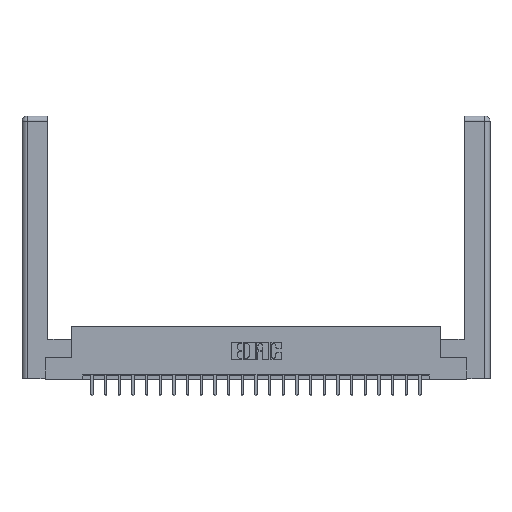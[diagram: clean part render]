
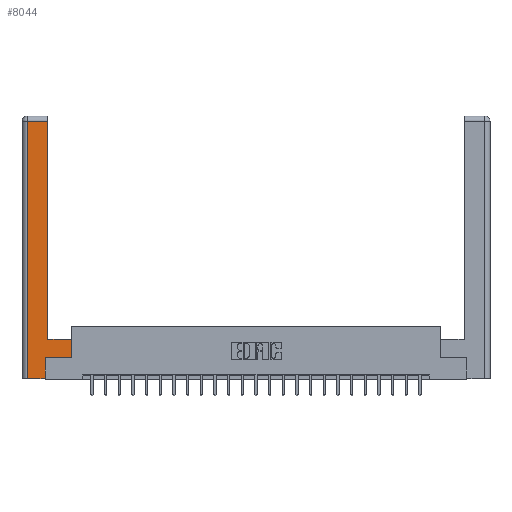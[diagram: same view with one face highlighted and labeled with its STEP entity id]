
A CAD part, top view. The second image highlights one B-rep face of the part: STEP entity #8044.
In plain terms, the highlighted planar face has unit normal (0, 0, 1).
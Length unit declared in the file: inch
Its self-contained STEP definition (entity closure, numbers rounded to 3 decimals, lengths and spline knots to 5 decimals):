
#282 = EDGE_LOOP ( 'NONE', ( #10034, #5375, #18630, #16974, #4671, #824, #2832, #15656 ) ) ;
#824 = ORIENTED_EDGE ( 'NONE', *, *, #4130, .T. ) ;
#983 = CARTESIAN_POINT ( 'NONE',  ( 0.0615, 0., 0. ) ) ;
#1534 = EDGE_CURVE ( 'NONE', #4164, #9989, #23469, .T. ) ;
#1827 = CARTESIAN_POINT ( 'NONE',  ( 0.295, 0.45, 0. ) ) ;
#1975 = FACE_OUTER_BOUND ( 'NONE', #282, .T. ) ;
#2264 = CARTESIAN_POINT ( 'NONE',  ( 0.565, 0.45, 0. ) ) ;
#2832 = ORIENTED_EDGE ( 'NONE', *, *, #22655, .T. ) ;
#2943 = CARTESIAN_POINT ( 'NONE',  ( 0., 0., 0. ) ) ;
#3510 = LINE ( 'NONE', #2264, #11119 ) ;
#4028 = CARTESIAN_POINT ( 'NONE',  ( 0.565, 0.245, 0. ) ) ;
#4130 = EDGE_CURVE ( 'NONE', #22083, #5999, #19548, .T. ) ;
#4164 = VERTEX_POINT ( 'NONE', #24257 ) ;
#4671 = ORIENTED_EDGE ( 'NONE', *, *, #22388, .T. ) ;
#4868 = VECTOR ( 'NONE', #6932, 39.37008 ) ;
#5162 = DIRECTION ( 'NONE',  ( 1., 0., 0. ) ) ;
#5306 = CARTESIAN_POINT ( 'NONE',  ( 0.0615, 2.94, 0. ) ) ;
#5375 = ORIENTED_EDGE ( 'NONE', *, *, #24340, .T. ) ;
#5926 = DIRECTION ( 'NONE',  ( 0., 1., 0. ) ) ;
#5999 = VERTEX_POINT ( 'NONE', #4028 ) ;
#6002 = VERTEX_POINT ( 'NONE', #6073 ) ;
#6073 = CARTESIAN_POINT ( 'NONE',  ( 0.295, 2.94, 0. ) ) ;
#6134 = VERTEX_POINT ( 'NONE', #21155 ) ;
#6441 = LINE ( 'NONE', #1827, #21457 ) ;
#6932 = DIRECTION ( 'NONE',  ( 1., 0., 0. ) ) ;
#7495 = DIRECTION ( 'NONE',  ( -1., 0., 0. ) ) ;
#7899 = AXIS2_PLACEMENT_3D ( 'NONE', #2943, #23398, #20022 ) ;
#8044 = ADVANCED_FACE ( 'NONE', ( #1975 ), #21701, .F. ) ;
#9989 = VERTEX_POINT ( 'NONE', #983 ) ;
#10034 = ORIENTED_EDGE ( 'NONE', *, *, #12761, .T. ) ;
#11119 = VECTOR ( 'NONE', #14353, 39.37008 ) ;
#11218 = CARTESIAN_POINT ( 'NONE',  ( 0.565, 0.245, 0. ) ) ;
#11517 = LINE ( 'NONE', #22686, #11844 ) ;
#11844 = VECTOR ( 'NONE', #5926, 39.37008 ) ;
#12761 = EDGE_CURVE ( 'NONE', #6134, #6002, #20354, .T. ) ;
#13144 = CARTESIAN_POINT ( 'NONE',  ( 0.265, 0., 0. ) ) ;
#13350 = LINE ( 'NONE', #5306, #18342 ) ;
#14319 = EDGE_CURVE ( 'NONE', #16274, #6134, #6441, .T. ) ;
#14353 = DIRECTION ( 'NONE',  ( 0., 1., 0. ) ) ;
#14760 = DIRECTION ( 'NONE',  ( -1., 0., 0. ) ) ;
#14783 = VECTOR ( 'NONE', #16453, 39.37008 ) ;
#14823 = CARTESIAN_POINT ( 'NONE',  ( 0.295, 3., 0. ) ) ;
#15433 = CARTESIAN_POINT ( 'NONE',  ( 0.565, 0.45, 0. ) ) ;
#15656 = ORIENTED_EDGE ( 'NONE', *, *, #14319, .T. ) ;
#16070 = VECTOR ( 'NONE', #5162, 39.37008 ) ;
#16274 = VERTEX_POINT ( 'NONE', #15433 ) ;
#16403 = CARTESIAN_POINT ( 'NONE',  ( 0.265, 0.245, 0. ) ) ;
#16453 = DIRECTION ( 'NONE',  ( 0., 1., 0. ) ) ;
#16974 = ORIENTED_EDGE ( 'NONE', *, *, #23736, .T. ) ;
#17693 = VERTEX_POINT ( 'NONE', #18665 ) ;
#18163 = VECTOR ( 'NONE', #23914, 39.37008 ) ;
#18342 = VECTOR ( 'NONE', #14760, 39.37008 ) ;
#18630 = ORIENTED_EDGE ( 'NONE', *, *, #1534, .T. ) ;
#18665 = CARTESIAN_POINT ( 'NONE',  ( 0.265, 0., 0. ) ) ;
#19548 = LINE ( 'NONE', #11218, #4868 ) ;
#20022 = DIRECTION ( 'NONE',  ( -1., 0., 0. ) ) ;
#20354 = LINE ( 'NONE', #14823, #14783 ) ;
#21155 = CARTESIAN_POINT ( 'NONE',  ( 0.295, 0.45, 0. ) ) ;
#21457 = VECTOR ( 'NONE', #7495, 39.37008 ) ;
#21701 = PLANE ( 'NONE',  #7899 ) ;
#22033 = CARTESIAN_POINT ( 'NONE',  ( 0.0615, 0., 0. ) ) ;
#22083 = VERTEX_POINT ( 'NONE', #16403 ) ;
#22388 = EDGE_CURVE ( 'NONE', #17693, #22083, #11517, .T. ) ;
#22503 = LINE ( 'NONE', #13144, #16070 ) ;
#22655 = EDGE_CURVE ( 'NONE', #5999, #16274, #3510, .T. ) ;
#22686 = CARTESIAN_POINT ( 'NONE',  ( 0.265, 0.245, 0. ) ) ;
#23398 = DIRECTION ( 'NONE',  ( 0., 0., -1. ) ) ;
#23469 = LINE ( 'NONE', #22033, #18163 ) ;
#23736 = EDGE_CURVE ( 'NONE', #9989, #17693, #22503, .T. ) ;
#23914 = DIRECTION ( 'NONE',  ( 0., -1., 0. ) ) ;
#24257 = CARTESIAN_POINT ( 'NONE',  ( 0.0615, 2.94, 0. ) ) ;
#24340 = EDGE_CURVE ( 'NONE', #6002, #4164, #13350, .T. ) ;
